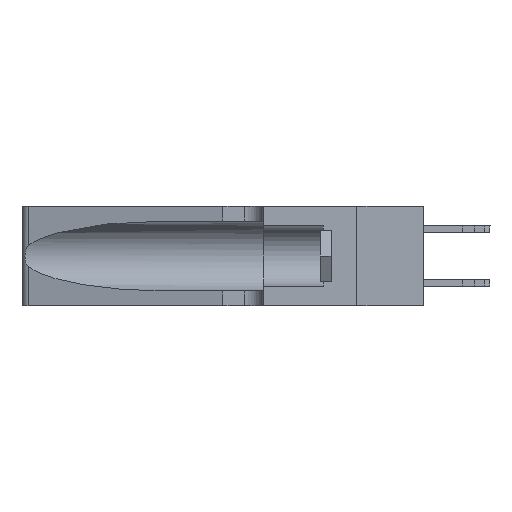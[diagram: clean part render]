
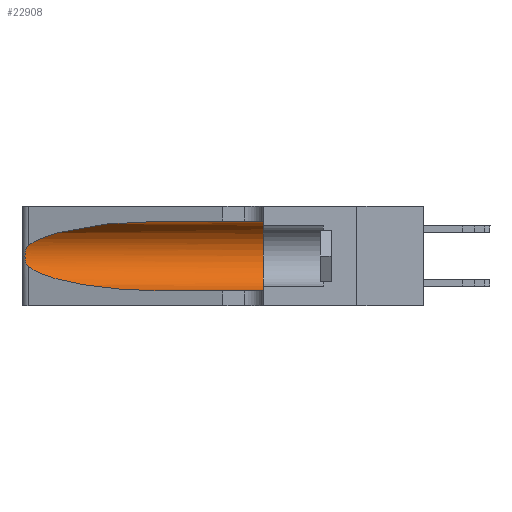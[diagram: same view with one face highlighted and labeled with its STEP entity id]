
A CAD part, left-side view. The second image highlights one B-rep face of the part: STEP entity #22908.
In plain terms, the highlighted cylindrical face has radius 3.308 mm (diameter 6.617 mm), a partial arc.
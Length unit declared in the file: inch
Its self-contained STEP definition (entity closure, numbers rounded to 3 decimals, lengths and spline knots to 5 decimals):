
#774 = AXIS2_PLACEMENT_3D ( 'NONE', #6077, #27972, #16941 ) ;
#2446 = CARTESIAN_POINT ( 'NONE',  ( 0.26018, 1.23835, 0.19895 ) ) ;
#2831 = CARTESIAN_POINT ( 'NONE',  ( 0.2373, 1.15595, 0.08982 ) ) ;
#3294 = ORIENTED_EDGE ( 'NONE', *, *, #3904, .T. ) ;
#3413 = CARTESIAN_POINT ( 'NONE',  ( 0.2373, 1.15595, 0.28018 ) ) ;
#3904 = EDGE_CURVE ( 'NONE', #9237, #20692, #29364, .T. ) ;
#5314 = CARTESIAN_POINT ( 'NONE',  ( 0.25639, 1.23184, 0.21858 ) ) ;
#5765 = ORIENTED_EDGE ( 'NONE', *, *, #30254, .T. ) ;
#5925 = CARTESIAN_POINT ( 'NONE',  ( 0.1305, 0.72297, 0.31525 ) ) ;
#5964 = LINE ( 'NONE', #25903, #6411 ) ;
#6077 = CARTESIAN_POINT ( 'NONE',  ( 0.1305, 1.61858, 0.185 ) ) ;
#6172 = CARTESIAN_POINT ( 'NONE',  ( 0.18966, 0.96281, 0.31525 ) ) ;
#6355 = ORIENTED_EDGE ( 'NONE', *, *, #30617, .T. ) ;
#6411 = VECTOR ( 'NONE', #12383, 39.37008 ) ;
#7811 = CARTESIAN_POINT ( 'NONE',  ( 0.25639, 1.23186, 0.15144 ) ) ;
#8067 = CARTESIAN_POINT ( 'NONE',  ( 0.1305, 0.72297, 0.05475 ) ) ;
#9237 = VERTEX_POINT ( 'NONE', #18087 ) ;
#9342 = CARTESIAN_POINT ( 'NONE',  ( 0.1305, 0.72297, 0.31525 ) ) ;
#9534 = VERTEX_POINT ( 'NONE', #30049 ) ;
#10359 =( BOUNDED_CURVE ( )  B_SPLINE_CURVE ( 3, ( #5925, #6172, #3413, #25112 ),
 .UNSPECIFIED., .F., .F. ) 
 B_SPLINE_CURVE_WITH_KNOTS ( ( 4, 4 ),
 ( 1.5708, 2.84003 ),
 .UNSPECIFIED. ) 
 CURVE ( )  GEOMETRIC_REPRESENTATION_ITEM ( )  RATIONAL_B_SPLINE_CURVE ( ( 1., 0.87, 0.87, 1. ) ) 
 REPRESENTATION_ITEM ( '' )  );
#10509 = CARTESIAN_POINT ( 'NONE',  ( 0.26017, 1.23833, 0.17102 ) ) ;
#10626 = CARTESIAN_POINT ( 'NONE',  ( 0.25487, 1.22718, 0.22369 ) ) ;
#11716 = DIRECTION ( 'NONE',  ( 0., -1., 0. ) ) ;
#12185 = AXIS2_PLACEMENT_3D ( 'NONE', #26387, #15357, #29098 ) ;
#12383 = DIRECTION ( 'NONE',  ( 0., -1., 0. ) ) ;
#12695 = FACE_OUTER_BOUND ( 'NONE', #26888, .T. ) ;
#12725 = CARTESIAN_POINT ( 'NONE',  ( 0.1305, 0.35, 0.31525 ) ) ;
#13220 = CARTESIAN_POINT ( 'NONE',  ( 0.25856, 1.23593, 0.16098 ) ) ;
#13521 = ORIENTED_EDGE ( 'NONE', *, *, #34852, .T. ) ;
#14317 = EDGE_CURVE ( 'NONE', #27332, #20692, #22894, .T. ) ;
#15357 = DIRECTION ( 'NONE',  ( 0., 1., 0. ) ) ;
#16071 = CARTESIAN_POINT ( 'NONE',  ( 0.25787, 1.23484, 0.2124 ) ) ;
#16941 = DIRECTION ( 'NONE',  ( 0., 0., -1. ) ) ;
#17406 = CARTESIAN_POINT ( 'NONE',  ( 0.1305, 0.35, 0.05475 ) ) ;
#18087 = CARTESIAN_POINT ( 'NONE',  ( 0.1305, 0.72297, 0.05475 ) ) ;
#18305 = CARTESIAN_POINT ( 'NONE',  ( 0.25854, 1.2359, 0.20912 ) ) ;
#18428 = CARTESIAN_POINT ( 'NONE',  ( 0.25789, 1.23486, 0.15765 ) ) ;
#18535 = CARTESIAN_POINT ( 'NONE',  ( 0.26075, 1.23896, 0.178 ) ) ;
#18600 =( BOUNDED_CURVE ( )  B_SPLINE_CURVE ( 3, ( #29603, #2831, #21923, #8067 ),
 .UNSPECIFIED., .F., .F. ) 
 B_SPLINE_CURVE_WITH_KNOTS ( ( 4, 4 ),
 ( 3.44316, 4.71239 ),
 .UNSPECIFIED. ) 
 CURVE ( )  GEOMETRIC_REPRESENTATION_ITEM ( )  RATIONAL_B_SPLINE_CURVE ( ( 1., 0.87, 0.87, 1. ) ) 
 REPRESENTATION_ITEM ( '' )  );
#18825 = ORIENTED_EDGE ( 'NONE', *, *, #28983, .F. ) ;
#19783 = CARTESIAN_POINT ( 'NONE',  ( 0.1305, 1.61858, 0.05475 ) ) ;
#20692 = VERTEX_POINT ( 'NONE', #17406 ) ;
#21923 = CARTESIAN_POINT ( 'NONE',  ( 0.18966, 0.96281, 0.05475 ) ) ;
#22894 = CIRCLE ( 'NONE', #12185, 0.13025 ) ;
#22908 = ADVANCED_FACE ( 'NONE', ( #12695 ), #26278, .F. ) ;
#25112 = CARTESIAN_POINT ( 'NONE',  ( 0.25487, 1.22718, 0.22369 ) ) ;
#25243 = CARTESIAN_POINT ( 'NONE',  ( 0.25487, 1.22718, 0.14631 ) ) ;
#25903 = CARTESIAN_POINT ( 'NONE',  ( 0.1305, 1.61858, 0.31525 ) ) ;
#26278 = CYLINDRICAL_SURFACE ( 'NONE', #774, 0.13025 ) ;
#26387 = CARTESIAN_POINT ( 'NONE',  ( 0.1305, 0.35, 0.185 ) ) ;
#26760 = CARTESIAN_POINT ( 'NONE',  ( 0.25555, 1.22993, 0.14849 ) ) ;
#26888 = EDGE_LOOP ( 'NONE', ( #5765, #6355, #13521, #3294, #31598, #18825 ) ) ;
#27297 = VECTOR ( 'NONE', #11716, 39.37008 ) ;
#27332 = VERTEX_POINT ( 'NONE', #12725 ) ;
#27972 = DIRECTION ( 'NONE',  ( 0., -1., 0. ) ) ;
#28216 = VERTEX_POINT ( 'NONE', #25243 ) ;
#28983 = EDGE_CURVE ( 'NONE', #32257, #27332, #5964, .T. ) ;
#29098 = DIRECTION ( 'NONE',  ( 0., 0., 1. ) ) ;
#29364 = LINE ( 'NONE', #19783, #27297 ) ;
#29460 = CARTESIAN_POINT ( 'NONE',  ( 0.25487, 1.22718, 0.14631 ) ) ;
#29603 = CARTESIAN_POINT ( 'NONE',  ( 0.25487, 1.22718, 0.14631 ) ) ;
#30049 = CARTESIAN_POINT ( 'NONE',  ( 0.25487, 1.22718, 0.22369 ) ) ;
#30254 = EDGE_CURVE ( 'NONE', #32257, #9534, #10359, .T. ) ;
#30617 = EDGE_CURVE ( 'NONE', #9534, #28216, #31191, .T. ) ;
#31191 = B_SPLINE_CURVE_WITH_KNOTS ( 'NONE', 3,
 ( #10626, #31811, #5314, #16071, #18305, #2446, #34521, #18535, #10509, #13220, #18428, #7811, #26760, #29460 ),
 .UNSPECIFIED., .F., .F.,
 ( 4, 2, 2, 2, 2, 2, 4 ),
 ( 0., 0.00027, 0.00053, 0.00107, 0.0016, 0.00187, 0.00214 ),
 .UNSPECIFIED. ) ;
#31598 = ORIENTED_EDGE ( 'NONE', *, *, #14317, .F. ) ;
#31811 = CARTESIAN_POINT ( 'NONE',  ( 0.25555, 1.22994, 0.2215 ) ) ;
#32257 = VERTEX_POINT ( 'NONE', #9342 ) ;
#34521 = CARTESIAN_POINT ( 'NONE',  ( 0.26075, 1.23896, 0.19203 ) ) ;
#34852 = EDGE_CURVE ( 'NONE', #28216, #9237, #18600, .T. ) ;
